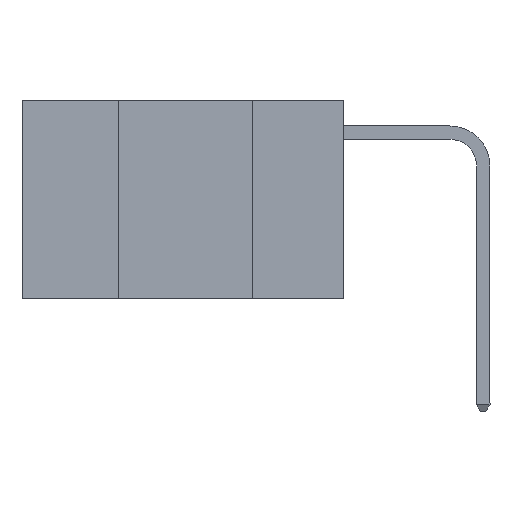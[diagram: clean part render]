
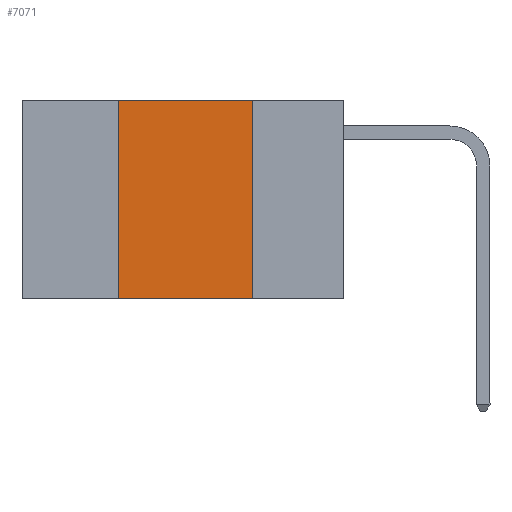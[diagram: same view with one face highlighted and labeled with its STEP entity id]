
A CAD part, left-side view. The second image highlights one B-rep face of the part: STEP entity #7071.
In plain terms, the highlighted planar face has unit normal (-1, 0, 0).
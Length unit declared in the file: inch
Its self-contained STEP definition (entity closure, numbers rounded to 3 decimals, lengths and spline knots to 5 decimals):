
#264 = CARTESIAN_POINT ( 'NONE',  ( 0., 0.6, 0. ) ) ;
#355 = VERTEX_POINT ( 'NONE', #4579 ) ;
#560 = CARTESIAN_POINT ( 'NONE',  ( 0., 0.42, 0. ) ) ;
#1089 = DIRECTION ( 'NONE',  ( 0., 0., 1. ) ) ;
#1890 = EDGE_CURVE ( 'NONE', #2206, #355, #8747, .T. ) ;
#2206 = VERTEX_POINT ( 'NONE', #8941 ) ;
#2326 = DIRECTION ( 'NONE',  ( 0., 0., -1. ) ) ;
#2435 = VECTOR ( 'NONE', #2326, 39.37008 ) ;
#2538 = LINE ( 'NONE', #8510, #2435 ) ;
#2614 = EDGE_CURVE ( 'NONE', #3800, #2206, #6617, .T. ) ;
#3338 = ORIENTED_EDGE ( 'NONE', *, *, #8831, .F. ) ;
#3446 = EDGE_CURVE ( 'NONE', #3800, #7124, #4651, .T. ) ;
#3465 = ORIENTED_EDGE ( 'NONE', *, *, #1890, .F. ) ;
#3800 = VERTEX_POINT ( 'NONE', #5296 ) ;
#3802 = ORIENTED_EDGE ( 'NONE', *, *, #2614, .F. ) ;
#4438 = ORIENTED_EDGE ( 'NONE', *, *, #3446, .T. ) ;
#4554 = EDGE_LOOP ( 'NONE', ( #3338, #3465, #3802, #4438 ) ) ;
#4579 = CARTESIAN_POINT ( 'NONE',  ( 0., 0.17, 0. ) ) ;
#4631 = VECTOR ( 'NONE', #7942, 39.37008 ) ;
#4651 = LINE ( 'NONE', #7984, #4631 ) ;
#5093 = CARTESIAN_POINT ( 'NONE',  ( 0., 0.17, -0.37 ) ) ;
#5296 = CARTESIAN_POINT ( 'NONE',  ( 0., 0.42, -0.37 ) ) ;
#5698 = CARTESIAN_POINT ( 'NONE',  ( 0., 0.6, 0. ) ) ;
#5731 = DIRECTION ( 'NONE',  ( 0., -1., 0. ) ) ;
#6045 = DIRECTION ( 'NONE',  ( 0., 0., -1. ) ) ;
#6560 = FACE_OUTER_BOUND ( 'NONE', #4554, .T. ) ;
#6617 = LINE ( 'NONE', #560, #6645 ) ;
#6645 = VECTOR ( 'NONE', #1089, 39.37008 ) ;
#7071 = ADVANCED_FACE ( 'NONE', ( #6560 ), #9921, .F. ) ;
#7124 = VERTEX_POINT ( 'NONE', #5093 ) ;
#7337 = AXIS2_PLACEMENT_3D ( 'NONE', #264, #9760, #6045 ) ;
#7942 = DIRECTION ( 'NONE',  ( 0., -1., 0. ) ) ;
#7984 = CARTESIAN_POINT ( 'NONE',  ( 0., 0.6, -0.37 ) ) ;
#8510 = CARTESIAN_POINT ( 'NONE',  ( 0., 0.17, 0. ) ) ;
#8747 = LINE ( 'NONE', #5698, #8790 ) ;
#8790 = VECTOR ( 'NONE', #5731, 39.37008 ) ;
#8831 = EDGE_CURVE ( 'NONE', #355, #7124, #2538, .T. ) ;
#8941 = CARTESIAN_POINT ( 'NONE',  ( 0., 0.42, 0. ) ) ;
#9760 = DIRECTION ( 'NONE',  ( 1., 0., 0. ) ) ;
#9921 = PLANE ( 'NONE',  #7337 ) ;
